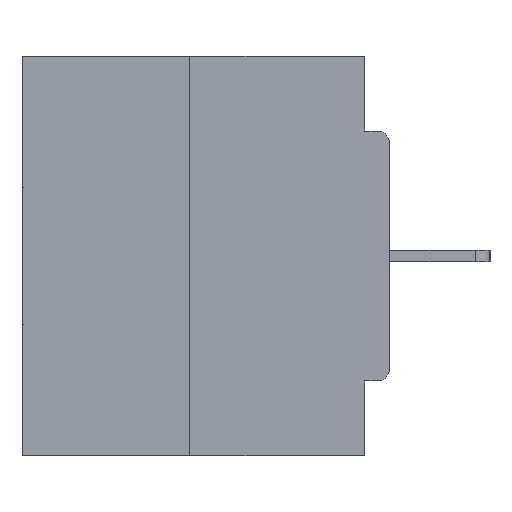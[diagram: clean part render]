
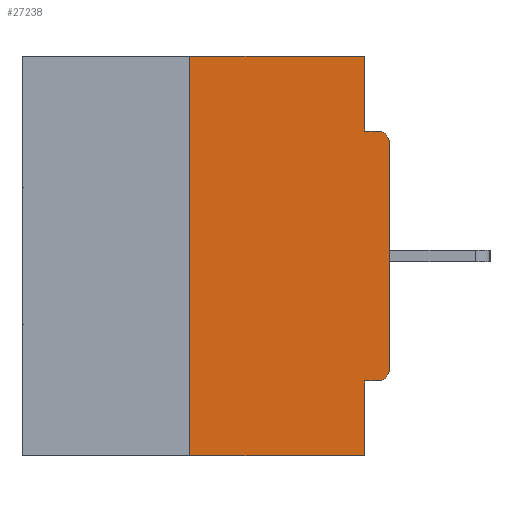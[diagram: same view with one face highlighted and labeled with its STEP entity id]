
A CAD part, left-side view. The second image highlights one B-rep face of the part: STEP entity #27238.
In plain terms, the highlighted planar face has unit normal (-1, 0, 0).
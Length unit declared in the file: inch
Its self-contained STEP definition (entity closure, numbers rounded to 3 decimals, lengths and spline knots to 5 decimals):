
#87 = DIRECTION ( 'NONE',  ( 0., -1., 0. ) ) ;
#357 = LINE ( 'NONE', #2771, #18025 ) ;
#632 = ORIENTED_EDGE ( 'NONE', *, *, #10357, .T. ) ;
#1206 = AXIS2_PLACEMENT_3D ( 'NONE', #13113, #16487, #10527 ) ;
#2771 = CARTESIAN_POINT ( 'NONE',  ( 0., 0., -0.4065 ) ) ;
#3002 = ORIENTED_EDGE ( 'NONE', *, *, #18808, .F. ) ;
#3429 = ORIENTED_EDGE ( 'NONE', *, *, #32313, .T. ) ;
#3630 = LINE ( 'NONE', #27289, #4248 ) ;
#4248 = VECTOR ( 'NONE', #24397, 39.37008 ) ;
#4269 = PLANE ( 'NONE',  #27658 ) ;
#4710 = VERTEX_POINT ( 'NONE', #6534 ) ;
#5351 = VECTOR ( 'NONE', #87, 39.37008 ) ;
#5379 = EDGE_CURVE ( 'NONE', #26031, #4710, #18794, .T. ) ;
#5911 = CARTESIAN_POINT ( 'NONE',  ( 0., 0.015, -0.3915 ) ) ;
#6174 = ORIENTED_EDGE ( 'NONE', *, *, #18127, .F. ) ;
#6534 = CARTESIAN_POINT ( 'NONE',  ( 0., 0.031, -0.5 ) ) ;
#7666 = CARTESIAN_POINT ( 'NONE',  ( 0., 0., -0.0935 ) ) ;
#8263 = EDGE_CURVE ( 'NONE', #17118, #14111, #33711, .T. ) ;
#8333 = DIRECTION ( 'NONE',  ( 0., -1., 0. ) ) ;
#8648 = CARTESIAN_POINT ( 'NONE',  ( 0., 0.25, 0. ) ) ;
#8737 = VERTEX_POINT ( 'NONE', #12886 ) ;
#9715 = CARTESIAN_POINT ( 'NONE',  ( 0., 0.031, 0. ) ) ;
#9858 = EDGE_CURVE ( 'NONE', #14111, #27389, #20696, .T. ) ;
#9948 = DIRECTION ( 'NONE',  ( 0., -1., 0. ) ) ;
#10265 = CARTESIAN_POINT ( 'NONE',  ( 0., 0.25, -0.5 ) ) ;
#10357 = EDGE_CURVE ( 'NONE', #8737, #27389, #31853, .T. ) ;
#10527 = DIRECTION ( 'NONE',  ( 0., 0., -1. ) ) ;
#10635 = LINE ( 'NONE', #20773, #15026 ) ;
#11303 = ORIENTED_EDGE ( 'NONE', *, *, #31731, .T. ) ;
#12519 = DIRECTION ( 'NONE',  ( 0., 0., -1. ) ) ;
#12528 = CARTESIAN_POINT ( 'NONE',  ( 0., 0.031, -0.4065 ) ) ;
#12886 = CARTESIAN_POINT ( 'NONE',  ( 0., 0., -0.1085 ) ) ;
#13113 = CARTESIAN_POINT ( 'NONE',  ( 0., 0.015, -0.1085 ) ) ;
#13411 = DIRECTION ( 'NONE',  ( 0., 1., 0. ) ) ;
#14111 = VERTEX_POINT ( 'NONE', #27401 ) ;
#14589 = DIRECTION ( 'NONE',  ( 1., 0., 0. ) ) ;
#15026 = VECTOR ( 'NONE', #31553, 39.37008 ) ;
#15042 = DIRECTION ( 'NONE',  ( 0., 0., -1. ) ) ;
#16266 = CIRCLE ( 'NONE', #17350, 0.015 ) ;
#16398 = CARTESIAN_POINT ( 'NONE',  ( 0., 0.46, -0.5 ) ) ;
#16487 = DIRECTION ( 'NONE',  ( -1., 0., 0. ) ) ;
#17118 = VERTEX_POINT ( 'NONE', #32882 ) ;
#17350 = AXIS2_PLACEMENT_3D ( 'NONE', #5911, #21006, #31460 ) ;
#17467 = VECTOR ( 'NONE', #30399, 39.37008 ) ;
#17824 = EDGE_CURVE ( 'NONE', #23458, #28511, #357, .T. ) ;
#17887 = ORIENTED_EDGE ( 'NONE', *, *, #9858, .F. ) ;
#18025 = VECTOR ( 'NONE', #13411, 39.37008 ) ;
#18127 = EDGE_CURVE ( 'NONE', #18573, #17118, #22989, .T. ) ;
#18573 = VERTEX_POINT ( 'NONE', #8648 ) ;
#18674 = CARTESIAN_POINT ( 'NONE',  ( 0., 0.015, -0.4065 ) ) ;
#18794 = LINE ( 'NONE', #16398, #5351 ) ;
#18808 = EDGE_CURVE ( 'NONE', #26031, #18573, #19784, .T. ) ;
#19784 = LINE ( 'NONE', #30234, #17467 ) ;
#20333 = VECTOR ( 'NONE', #8333, 39.37008 ) ;
#20696 = LINE ( 'NONE', #7666, #20333 ) ;
#20757 = VECTOR ( 'NONE', #9948, 39.37008 ) ;
#20773 = CARTESIAN_POINT ( 'NONE',  ( 0., 0.031, -0.5 ) ) ;
#21006 = DIRECTION ( 'NONE',  ( -1., 0., 0. ) ) ;
#21936 = ORIENTED_EDGE ( 'NONE', *, *, #25596, .F. ) ;
#22989 = LINE ( 'NONE', #33447, #20757 ) ;
#23458 = VERTEX_POINT ( 'NONE', #18674 ) ;
#23629 = CARTESIAN_POINT ( 'NONE',  ( 0., 0.015, -0.0935 ) ) ;
#24397 = DIRECTION ( 'NONE',  ( 0., 0., 1. ) ) ;
#24640 = ORIENTED_EDGE ( 'NONE', *, *, #8263, .F. ) ;
#25259 = CARTESIAN_POINT ( 'NONE',  ( 0., 0., -0.3915 ) ) ;
#25555 = CARTESIAN_POINT ( 'NONE',  ( 0., 0.46, 0. ) ) ;
#25596 = EDGE_CURVE ( 'NONE', #28511, #4710, #10635, .T. ) ;
#26031 = VERTEX_POINT ( 'NONE', #10265 ) ;
#26774 = ORIENTED_EDGE ( 'NONE', *, *, #17824, .F. ) ;
#27238 = ADVANCED_FACE ( 'NONE', ( #30329 ), #4269, .F. ) ;
#27272 = ORIENTED_EDGE ( 'NONE', *, *, #5379, .T. ) ;
#27289 = CARTESIAN_POINT ( 'NONE',  ( 0., 0., 0. ) ) ;
#27389 = VERTEX_POINT ( 'NONE', #23629 ) ;
#27401 = CARTESIAN_POINT ( 'NONE',  ( 0., 0.031, -0.0935 ) ) ;
#27658 = AXIS2_PLACEMENT_3D ( 'NONE', #25555, #14589, #12519 ) ;
#28511 = VERTEX_POINT ( 'NONE', #12528 ) ;
#29077 = VECTOR ( 'NONE', #15042, 39.37008 ) ;
#29913 = EDGE_LOOP ( 'NONE', ( #6174, #3002, #27272, #21936, #26774, #11303, #3429, #632, #17887, #24640 ) ) ;
#30234 = CARTESIAN_POINT ( 'NONE',  ( 0., 0.25, 0. ) ) ;
#30329 = FACE_OUTER_BOUND ( 'NONE', #29913, .T. ) ;
#30399 = DIRECTION ( 'NONE',  ( 0., 0., 1. ) ) ;
#31460 = DIRECTION ( 'NONE',  ( 0., 0., -1. ) ) ;
#31553 = DIRECTION ( 'NONE',  ( 0., 0., -1. ) ) ;
#31731 = EDGE_CURVE ( 'NONE', #23458, #32448, #16266, .T. ) ;
#31853 = CIRCLE ( 'NONE', #1206, 0.015 ) ;
#32313 = EDGE_CURVE ( 'NONE', #32448, #8737, #3630, .T. ) ;
#32448 = VERTEX_POINT ( 'NONE', #25259 ) ;
#32882 = CARTESIAN_POINT ( 'NONE',  ( 0., 0.031, 0. ) ) ;
#33447 = CARTESIAN_POINT ( 'NONE',  ( 0., 0.46, 0. ) ) ;
#33711 = LINE ( 'NONE', #9715, #29077 ) ;
